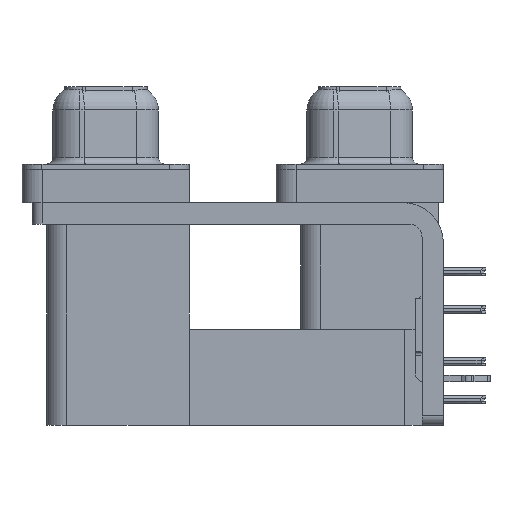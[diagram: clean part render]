
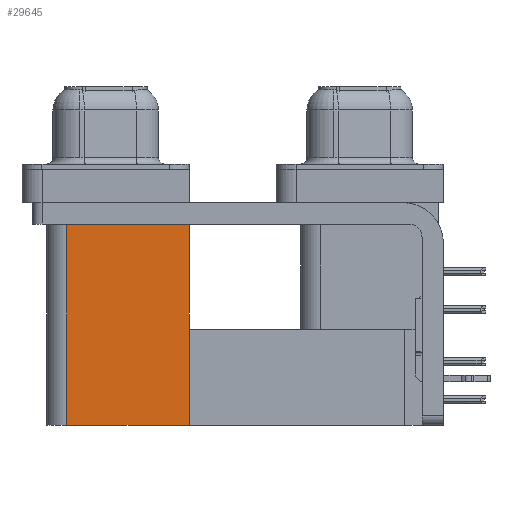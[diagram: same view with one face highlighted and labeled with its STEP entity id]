
A CAD part, left-side view. The second image highlights one B-rep face of the part: STEP entity #29645.
In plain terms, the highlighted planar face has unit normal (-1, 0, 0).
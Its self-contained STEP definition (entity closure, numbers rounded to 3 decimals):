
#1238 = VECTOR ( 'NONE', #43225, 1000. ) ;
#2492 = CARTESIAN_POINT ( 'NONE',  ( 3.765, 12.775, -19.2 ) ) ;
#4343 = CARTESIAN_POINT ( 'NONE',  ( 3.765, 21.975, -19.2 ) ) ;
#4530 = CARTESIAN_POINT ( 'NONE',  ( 3.765, 12.775, -2.5 ) ) ;
#6165 = LINE ( 'NONE', #25151, #34455 ) ;
#6341 = VECTOR ( 'NONE', #45524, 1000. ) ;
#8315 = EDGE_CURVE ( 'NONE', #30588, #15655, #45022, .T. ) ;
#9739 = CARTESIAN_POINT ( 'NONE',  ( 3.765, 12.775, -2.5 ) ) ;
#9832 = ORIENTED_EDGE ( 'NONE', *, *, #8315, .T. ) ;
#10185 = CARTESIAN_POINT ( 'NONE',  ( 3.765, 12.775, -19.2 ) ) ;
#13069 = EDGE_LOOP ( 'NONE', ( #40919, #34268, #43273, #9832 ) ) ;
#13300 = DIRECTION ( 'NONE',  ( 0., 0., -1. ) ) ;
#13492 = LINE ( 'NONE', #42900, #42215 ) ;
#14593 = LINE ( 'NONE', #4530, #1238 ) ;
#15655 = VERTEX_POINT ( 'NONE', #9739 ) ;
#20206 = AXIS2_PLACEMENT_3D ( 'NONE', #2492, #48390, #13300 ) ;
#25151 = CARTESIAN_POINT ( 'NONE',  ( 3.765, 12.775, -19.2 ) ) ;
#25415 = CARTESIAN_POINT ( 'NONE',  ( 3.765, 12.775, -19.2 ) ) ;
#25740 = CARTESIAN_POINT ( 'NONE',  ( 3.765, 21.975, -2.5 ) ) ;
#25847 = FACE_OUTER_BOUND ( 'NONE', #13069, .T. ) ;
#28242 = EDGE_CURVE ( 'NONE', #29440, #36570, #13492, .T. ) ;
#28974 = DIRECTION ( 'NONE',  ( 0., 1., 0. ) ) ;
#29440 = VERTEX_POINT ( 'NONE', #4343 ) ;
#29645 = ADVANCED_FACE ( 'NONE', ( #25847 ), #37627, .F. ) ;
#30588 = VERTEX_POINT ( 'NONE', #25415 ) ;
#30627 = DIRECTION ( 'NONE',  ( 0., 0., 1. ) ) ;
#34268 = ORIENTED_EDGE ( 'NONE', *, *, #28242, .F. ) ;
#34455 = VECTOR ( 'NONE', #28974, 1000. ) ;
#35418 = EDGE_CURVE ( 'NONE', #30588, #29440, #6165, .T. ) ;
#36570 = VERTEX_POINT ( 'NONE', #25740 ) ;
#37627 = PLANE ( 'NONE',  #20206 ) ;
#40919 = ORIENTED_EDGE ( 'NONE', *, *, #41239, .T. ) ;
#41239 = EDGE_CURVE ( 'NONE', #15655, #36570, #14593, .T. ) ;
#42215 = VECTOR ( 'NONE', #30627, 1000. ) ;
#42900 = CARTESIAN_POINT ( 'NONE',  ( 3.765, 21.975, -19.2 ) ) ;
#43225 = DIRECTION ( 'NONE',  ( 0., 1., 0. ) ) ;
#43273 = ORIENTED_EDGE ( 'NONE', *, *, #35418, .F. ) ;
#45022 = LINE ( 'NONE', #10185, #6341 ) ;
#45524 = DIRECTION ( 'NONE',  ( 0., 0., 1. ) ) ;
#48390 = DIRECTION ( 'NONE',  ( 1., 0., 0. ) ) ;
